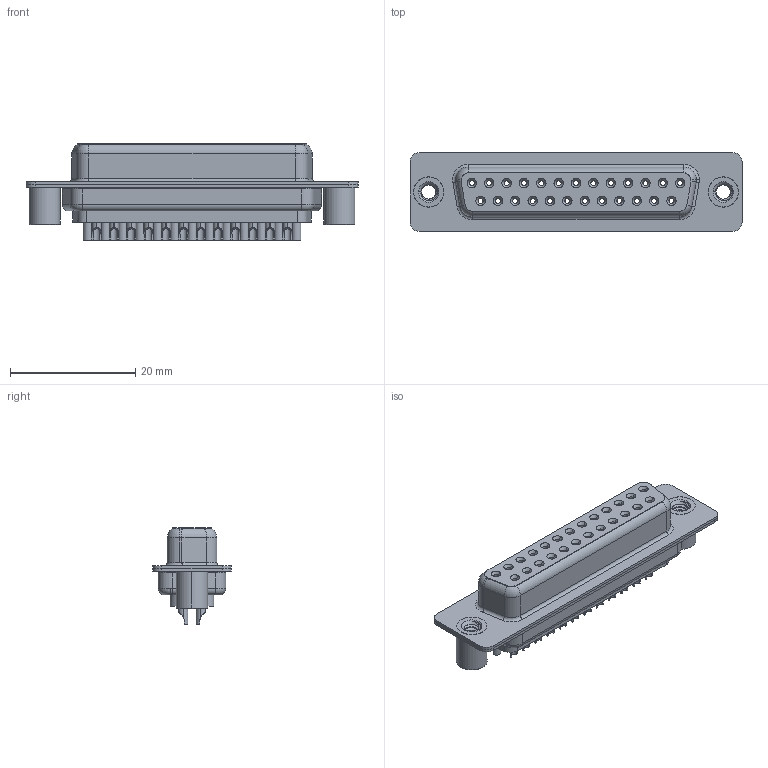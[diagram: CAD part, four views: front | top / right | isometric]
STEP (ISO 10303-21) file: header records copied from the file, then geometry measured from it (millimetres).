
FILE_DESCRIPTION (( 'STEP AP203' ), '1' );
FILE_NAME ('628-025-322-249.STEP', '2020-07-14T13:57:04', ( '' ), ( '' ), 'SwSTEP 2.0', 'SolidWorks 2020', '' );
FILE_SCHEMA (( 'CONFIG_CONTROL_DESIGN' ));
Length unit declared in the file: millimetre
Products named in the file (7): 628 Contact Row 1_22L; 628 Contact Row 2_22L; 628 Shell Front_25 Contacts; 628-025-322-249; 628 Shell Rear_25 Contacts; 628 4-40 Threaded Standoff BS; 628 Housing_25 LP
Assembly tree (30 placements, depth 2):
  628-025-322-249
    628 Housing_25 LP
    628 Shell Front_25 Contacts
    628 Shell Rear_25 Contacts
    628 Contact Row 1_22L  x13
    628 Contact Row 2_22L  x12
    628 4-40 Threaded Standoff BS  x2
Bounding box: 53 x 12.6 x 15.35 mm (x, y, z)
Volume: 3941 mm3; surface area: 9580.3 mm2
Topology: 30 solids, 30 shells, 2526 faces, 6399 edges, 4019 vertices
Faces by surface type: cylinder 782, plane 592, torus 507, bspline 506, cone 139
Entity records: 25978 total; most frequent: CARTESIAN_POINT 7417, DIRECTION 3791, ORIENTED_EDGE 3464, EDGE_CURVE 1732, AXIS2_PLACEMENT_3D 1586, VERTEX_POINT 1094, EDGE_LOOP 882, CIRCLE 862
